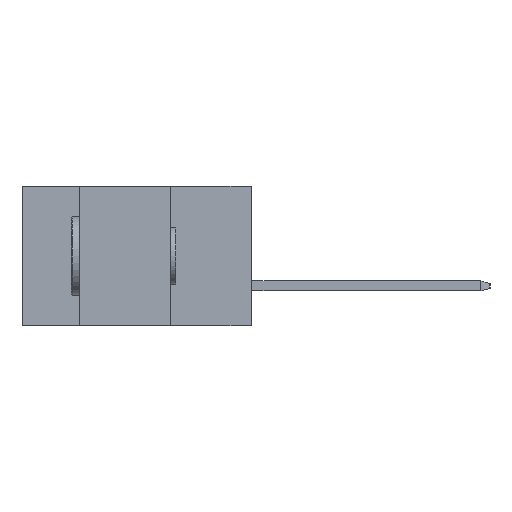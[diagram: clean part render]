
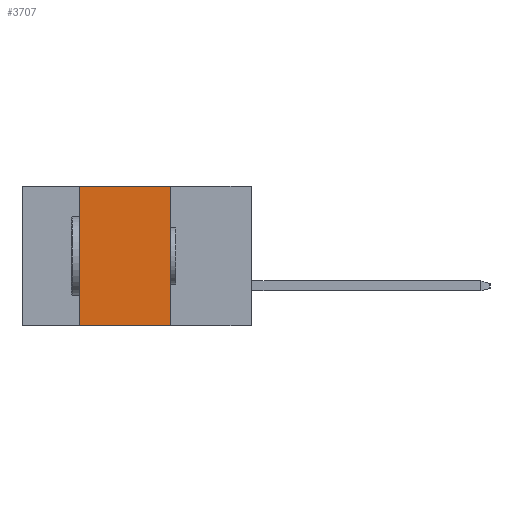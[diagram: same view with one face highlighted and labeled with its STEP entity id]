
A CAD part, left-side view. The second image highlights one B-rep face of the part: STEP entity #3707.
In plain terms, the highlighted planar face has unit normal (-1, 0, 0).
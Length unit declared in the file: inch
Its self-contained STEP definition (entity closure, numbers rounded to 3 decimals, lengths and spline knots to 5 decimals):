
#188 = EDGE_CURVE ( 'NONE', #3724, #4173, #7330, .T. ) ;
#214 = ORIENTED_EDGE ( 'NONE', *, *, #3281, .F. ) ;
#1715 = LINE ( 'NONE', #3867, #10281 ) ;
#1756 = ORIENTED_EDGE ( 'NONE', *, *, #188, .F. ) ;
#3175 = VERTEX_POINT ( 'NONE', #3936 ) ;
#3281 = EDGE_CURVE ( 'NONE', #3175, #3724, #1715, .T. ) ;
#3707 = ADVANCED_FACE ( 'NONE', ( #6811 ), #9967, .F. ) ;
#3724 = VERTEX_POINT ( 'NONE', #9098 ) ;
#3867 = CARTESIAN_POINT ( 'NONE',  ( 0., 0.54, -0.437 ) ) ;
#3933 = CARTESIAN_POINT ( 'NONE',  ( 0., 0.72, -0.437 ) ) ;
#3936 = CARTESIAN_POINT ( 'NONE',  ( 0., 0.54, -0.437 ) ) ;
#3978 = LINE ( 'NONE', #8211, #7486 ) ;
#4173 = VERTEX_POINT ( 'NONE', #10533 ) ;
#4210 = EDGE_CURVE ( 'NONE', #4173, #9051, #3978, .T. ) ;
#4455 = ORIENTED_EDGE ( 'NONE', *, *, #7555, .T. ) ;
#6254 = CARTESIAN_POINT ( 'NONE',  ( 0., 0.72, 0. ) ) ;
#6811 = FACE_OUTER_BOUND ( 'NONE', #12353, .T. ) ;
#7143 = VECTOR ( 'NONE', #10351, 39.37008 ) ;
#7330 = LINE ( 'NONE', #6254, #7143 ) ;
#7486 = VECTOR ( 'NONE', #11298, 39.37008 ) ;
#7555 = EDGE_CURVE ( 'NONE', #3175, #9051, #13155, .T. ) ;
#7825 = DIRECTION ( 'NONE',  ( 1., 0., 0. ) ) ;
#7850 = CARTESIAN_POINT ( 'NONE',  ( 0., 0.254, -0.437 ) ) ;
#8039 = DIRECTION ( 'NONE',  ( 0., -1., 0. ) ) ;
#8211 = CARTESIAN_POINT ( 'NONE',  ( 0., 0.254, -0.437 ) ) ;
#9051 = VERTEX_POINT ( 'NONE', #7850 ) ;
#9098 = CARTESIAN_POINT ( 'NONE',  ( 0., 0.54, 0. ) ) ;
#9916 = DIRECTION ( 'NONE',  ( 0., 0., 1. ) ) ;
#9967 = PLANE ( 'NONE',  #12856 ) ;
#10105 = DIRECTION ( 'NONE',  ( 0., 0., -1. ) ) ;
#10281 = VECTOR ( 'NONE', #9916, 39.37008 ) ;
#10351 = DIRECTION ( 'NONE',  ( 0., -1., 0. ) ) ;
#10533 = CARTESIAN_POINT ( 'NONE',  ( 0., 0.254, 0. ) ) ;
#11298 = DIRECTION ( 'NONE',  ( 0., 0., -1. ) ) ;
#11851 = CARTESIAN_POINT ( 'NONE',  ( 0., 0.72, 0. ) ) ;
#12353 = EDGE_LOOP ( 'NONE', ( #12927, #1756, #214, #4455 ) ) ;
#12382 = VECTOR ( 'NONE', #8039, 39.37008 ) ;
#12856 = AXIS2_PLACEMENT_3D ( 'NONE', #11851, #7825, #10105 ) ;
#12927 = ORIENTED_EDGE ( 'NONE', *, *, #4210, .F. ) ;
#13155 = LINE ( 'NONE', #3933, #12382 ) ;
